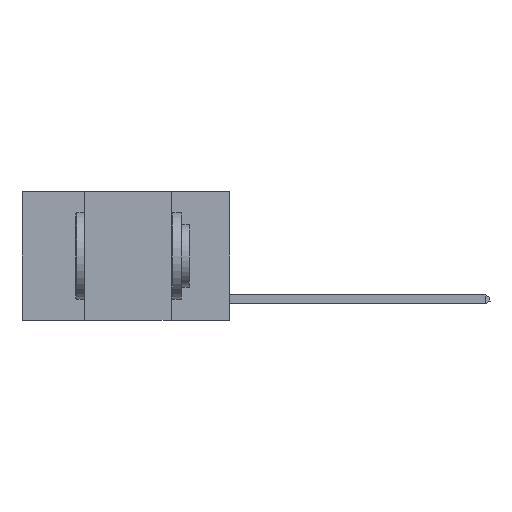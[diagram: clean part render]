
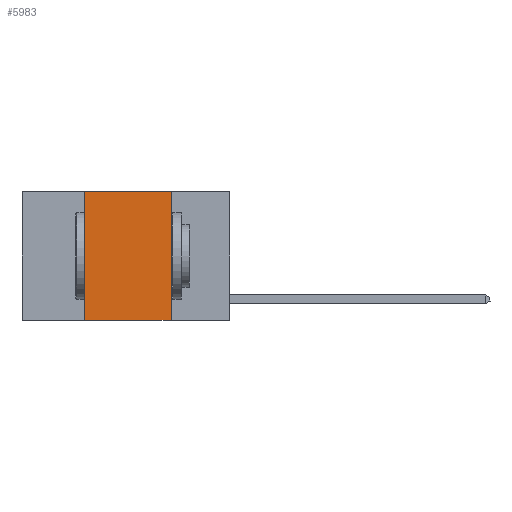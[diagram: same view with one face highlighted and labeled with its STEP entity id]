
A CAD part, left-side view. The second image highlights one B-rep face of the part: STEP entity #5983.
In plain terms, the highlighted planar face has unit normal (-1, 0, 0).
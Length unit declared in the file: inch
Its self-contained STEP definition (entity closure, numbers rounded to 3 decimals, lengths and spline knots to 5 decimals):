
#939 = ORIENTED_EDGE ( 'NONE', *, *, #4048, .T. ) ;
#1613 = EDGE_LOOP ( 'NONE', ( #15797, #21581, #13549, #939 ) ) ;
#1943 = CARTESIAN_POINT ( 'NONE',  ( 0., 0.42, 0. ) ) ;
#2706 = CARTESIAN_POINT ( 'NONE',  ( 0., 0.17, 0. ) ) ;
#3327 = VERTEX_POINT ( 'NONE', #18263 ) ;
#4048 = EDGE_CURVE ( 'NONE', #19809, #16994, #19774, .T. ) ;
#5632 = DIRECTION ( 'NONE',  ( 0., 0., 1. ) ) ;
#5983 = ADVANCED_FACE ( 'NONE', ( #16045 ), #23269, .F. ) ;
#6628 = VERTEX_POINT ( 'NONE', #2706 ) ;
#6767 = LINE ( 'NONE', #19674, #9991 ) ;
#6799 = LINE ( 'NONE', #15937, #16568 ) ;
#7015 = CARTESIAN_POINT ( 'NONE',  ( 0., 0.6, 0. ) ) ;
#8082 = AXIS2_PLACEMENT_3D ( 'NONE', #7015, #14250, #12830 ) ;
#8400 = DIRECTION ( 'NONE',  ( 0., -1., 0. ) ) ;
#9991 = VECTOR ( 'NONE', #17666, 39.37008 ) ;
#10754 = CARTESIAN_POINT ( 'NONE',  ( 0., 0.6, -0.37 ) ) ;
#12830 = DIRECTION ( 'NONE',  ( 0., 0., -1. ) ) ;
#12981 = EDGE_CURVE ( 'NONE', #19809, #3327, #14730, .T. ) ;
#13549 = ORIENTED_EDGE ( 'NONE', *, *, #12981, .F. ) ;
#14038 = DIRECTION ( 'NONE',  ( 0., -1., 0. ) ) ;
#14130 = CARTESIAN_POINT ( 'NONE',  ( 0., 0.17, -0.37 ) ) ;
#14250 = DIRECTION ( 'NONE',  ( 1., 0., 0. ) ) ;
#14730 = LINE ( 'NONE', #1943, #16905 ) ;
#15199 = EDGE_CURVE ( 'NONE', #3327, #6628, #6799, .T. ) ;
#15797 = ORIENTED_EDGE ( 'NONE', *, *, #21070, .F. ) ;
#15937 = CARTESIAN_POINT ( 'NONE',  ( 0., 0.6, 0. ) ) ;
#16045 = FACE_OUTER_BOUND ( 'NONE', #1613, .T. ) ;
#16322 = CARTESIAN_POINT ( 'NONE',  ( 0., 0.42, -0.37 ) ) ;
#16568 = VECTOR ( 'NONE', #14038, 39.37008 ) ;
#16905 = VECTOR ( 'NONE', #5632, 39.37008 ) ;
#16994 = VERTEX_POINT ( 'NONE', #14130 ) ;
#17361 = VECTOR ( 'NONE', #8400, 39.37008 ) ;
#17666 = DIRECTION ( 'NONE',  ( 0., 0., -1. ) ) ;
#18263 = CARTESIAN_POINT ( 'NONE',  ( 0., 0.42, 0. ) ) ;
#19674 = CARTESIAN_POINT ( 'NONE',  ( 0., 0.17, 0. ) ) ;
#19774 = LINE ( 'NONE', #10754, #17361 ) ;
#19809 = VERTEX_POINT ( 'NONE', #16322 ) ;
#21070 = EDGE_CURVE ( 'NONE', #6628, #16994, #6767, .T. ) ;
#21581 = ORIENTED_EDGE ( 'NONE', *, *, #15199, .F. ) ;
#23269 = PLANE ( 'NONE',  #8082 ) ;
